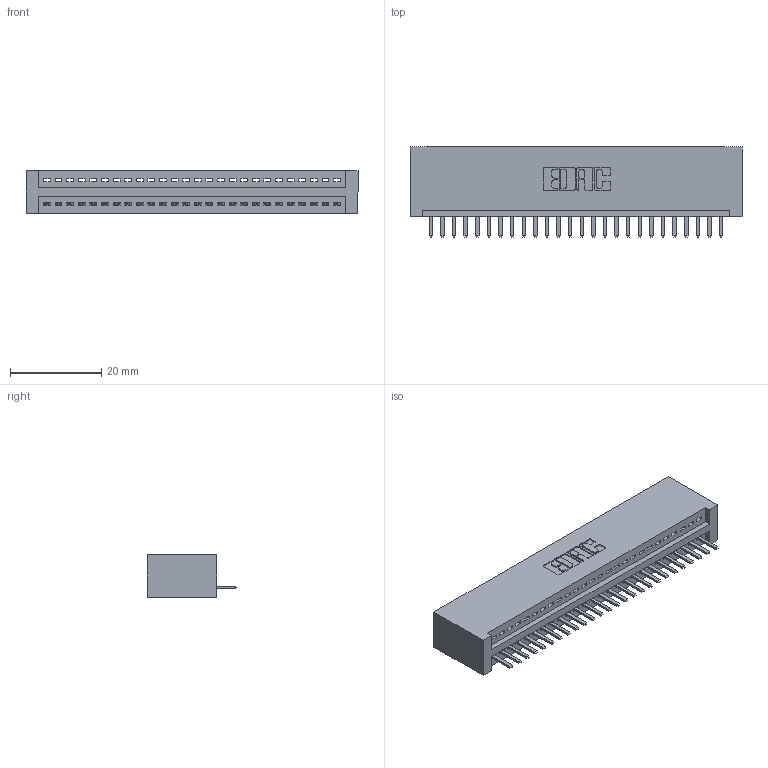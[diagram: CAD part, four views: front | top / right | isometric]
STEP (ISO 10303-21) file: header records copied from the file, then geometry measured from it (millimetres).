
FILE_DESCRIPTION (( 'STEP AP203' ), '1' );
FILE_NAME ('345-026-520-101.STEP', '2018-08-21T23:32:38', ( '' ), ( '' ), 'SwSTEP 2.0', 'SolidWorks 2016', '' );
FILE_SCHEMA (( 'CONFIG_CONTROL_DESIGN' ));
Length unit declared in the file: inch
Products named in the file (3): 345-026-520-101; 345 Part_No Mounting Lugs; 345-292-001_345-293-120
Assembly tree (27 placements, depth 2):
  345-026-520-101
    345 Part_No Mounting Lugs
    345-292-001_345-293-120  x26
Bounding box: 72.64 x 19.68 x 9.4 mm (x, y, z)
Volume: 7278.3 mm3; surface area: 9400.2 mm2
Topology: 27 solids, 27 shells, 1730 faces, 5101 edges, 3330 vertices
Faces by surface type: plane 1168, cylinder 562
Entity records: 21559 total; most frequent: CARTESIAN_POINT 3754, ORIENTED_EDGE 3702, DIRECTION 3283, EDGE_CURVE 1851, VECTOR 1619, LINE 1619, VERTEX_POINT 1230, AXIS2_PLACEMENT_3D 832
